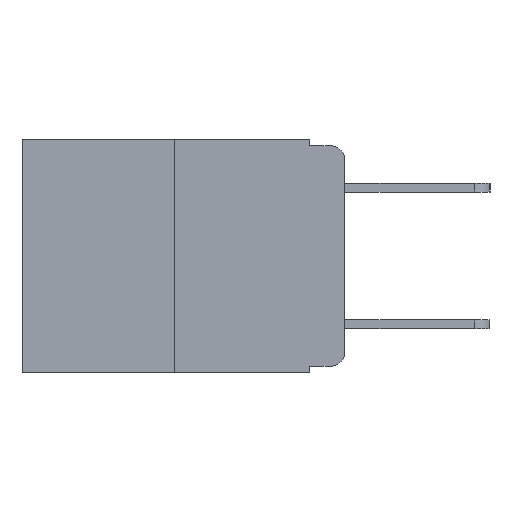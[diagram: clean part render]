
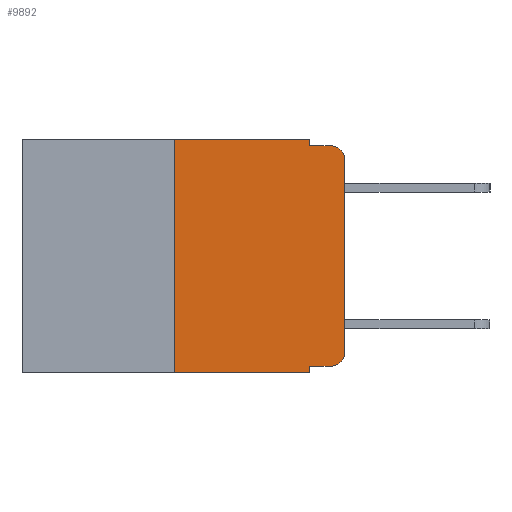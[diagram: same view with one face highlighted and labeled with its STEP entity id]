
A CAD part, left-side view. The second image highlights one B-rep face of the part: STEP entity #9892.
In plain terms, the highlighted planar face has unit normal (-1, 0, 0).
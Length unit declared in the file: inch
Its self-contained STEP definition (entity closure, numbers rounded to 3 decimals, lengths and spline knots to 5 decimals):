
#5 = DIRECTION ( 'NONE',  ( -1., 0., 0. ) ) ;
#24 = LINE ( 'NONE', #9948, #9604 ) ;
#371 = ORIENTED_EDGE ( 'NONE', *, *, #2360, .T. ) ;
#423 = CARTESIAN_POINT ( 'NONE',  ( 0., 0.051, -0.01 ) ) ;
#494 = VERTEX_POINT ( 'NONE', #6020 ) ;
#500 = LINE ( 'NONE', #2824, #9484 ) ;
#669 = VERTEX_POINT ( 'NONE', #9524 ) ;
#785 = LINE ( 'NONE', #10583, #5287 ) ;
#791 = CARTESIAN_POINT ( 'NONE',  ( 0., 0.25, 0. ) ) ;
#915 = VERTEX_POINT ( 'NONE', #4811 ) ;
#1352 = EDGE_CURVE ( 'NONE', #6785, #8225, #785, .T. ) ;
#1600 = EDGE_CURVE ( 'NONE', #3743, #2445, #8336, .T. ) ;
#1873 = ORIENTED_EDGE ( 'NONE', *, *, #1600, .T. ) ;
#1951 = DIRECTION ( 'NONE',  ( 0., -1., 0. ) ) ;
#1996 = CARTESIAN_POINT ( 'NONE',  ( 0., 0.051, -0.333 ) ) ;
#2031 = VERTEX_POINT ( 'NONE', #7292 ) ;
#2129 = LINE ( 'NONE', #4757, #11149 ) ;
#2158 = ORIENTED_EDGE ( 'NONE', *, *, #7004, .T. ) ;
#2360 = EDGE_CURVE ( 'NONE', #2031, #915, #2129, .T. ) ;
#2445 = VERTEX_POINT ( 'NONE', #4334 ) ;
#2824 = CARTESIAN_POINT ( 'NONE',  ( 0., 0., 0. ) ) ;
#2849 = EDGE_CURVE ( 'NONE', #669, #7589, #500, .T. ) ;
#3039 = DIRECTION ( 'NONE',  ( 0., 0., 1. ) ) ;
#3146 = DIRECTION ( 'NONE',  ( 0., -1., 0. ) ) ;
#3434 = ORIENTED_EDGE ( 'NONE', *, *, #6601, .F. ) ;
#3544 = PLANE ( 'NONE',  #4599 ) ;
#3712 = EDGE_LOOP ( 'NONE', ( #5486, #8665, #9512, #7982, #3840, #4403, #371, #3434, #1873, #2158 ) ) ;
#3743 = VERTEX_POINT ( 'NONE', #6516 ) ;
#3840 = ORIENTED_EDGE ( 'NONE', *, *, #3918, .F. ) ;
#3918 = EDGE_CURVE ( 'NONE', #494, #6785, #24, .T. ) ;
#3938 = CARTESIAN_POINT ( 'NONE',  ( 0., 0.051, 0. ) ) ;
#4020 = LINE ( 'NONE', #791, #8420 ) ;
#4027 = CIRCLE ( 'NONE', #5979, 0.02 ) ;
#4334 = CARTESIAN_POINT ( 'NONE',  ( 0., 0.02, -0.333 ) ) ;
#4403 = ORIENTED_EDGE ( 'NONE', *, *, #7378, .F. ) ;
#4441 = DIRECTION ( 'NONE',  ( 1., 0., 0. ) ) ;
#4599 = AXIS2_PLACEMENT_3D ( 'NONE', #11319, #4441, #10545 ) ;
#4757 = CARTESIAN_POINT ( 'NONE',  ( 0., 0.473, -0.343 ) ) ;
#4811 = CARTESIAN_POINT ( 'NONE',  ( 0., 0.051, -0.343 ) ) ;
#5054 = CARTESIAN_POINT ( 'NONE',  ( 0., 0.02, -0.03 ) ) ;
#5068 = FACE_OUTER_BOUND ( 'NONE', #3712, .T. ) ;
#5287 = VECTOR ( 'NONE', #7171, 39.37008 ) ;
#5456 = AXIS2_PLACEMENT_3D ( 'NONE', #5054, #11115, #5936 ) ;
#5457 = CARTESIAN_POINT ( 'NONE',  ( 0., 0.02, -0.313 ) ) ;
#5486 = ORIENTED_EDGE ( 'NONE', *, *, #2849, .T. ) ;
#5913 = VERTEX_POINT ( 'NONE', #9069 ) ;
#5936 = DIRECTION ( 'NONE',  ( 0., 0., -1. ) ) ;
#5979 = AXIS2_PLACEMENT_3D ( 'NONE', #5457, #5, #6356 ) ;
#6020 = CARTESIAN_POINT ( 'NONE',  ( 0., 0.25, 0. ) ) ;
#6171 = EDGE_CURVE ( 'NONE', #7589, #5913, #10599, .T. ) ;
#6356 = DIRECTION ( 'NONE',  ( 0., 0., -1. ) ) ;
#6516 = CARTESIAN_POINT ( 'NONE',  ( 0., 0.051, -0.333 ) ) ;
#6601 = EDGE_CURVE ( 'NONE', #3743, #915, #9007, .T. ) ;
#6785 = VERTEX_POINT ( 'NONE', #9536 ) ;
#7004 = EDGE_CURVE ( 'NONE', #2445, #669, #4027, .T. ) ;
#7171 = DIRECTION ( 'NONE',  ( 0., 0., -1. ) ) ;
#7292 = CARTESIAN_POINT ( 'NONE',  ( 0., 0.25, -0.343 ) ) ;
#7378 = EDGE_CURVE ( 'NONE', #2031, #494, #4020, .T. ) ;
#7585 = LINE ( 'NONE', #423, #10172 ) ;
#7589 = VERTEX_POINT ( 'NONE', #10127 ) ;
#7642 = DIRECTION ( 'NONE',  ( 0., -1., 0. ) ) ;
#7799 = CARTESIAN_POINT ( 'NONE',  ( 0., 0.051, -0.01 ) ) ;
#7982 = ORIENTED_EDGE ( 'NONE', *, *, #1352, .F. ) ;
#8153 = EDGE_CURVE ( 'NONE', #8225, #5913, #7585, .T. ) ;
#8225 = VERTEX_POINT ( 'NONE', #7799 ) ;
#8336 = LINE ( 'NONE', #1996, #10380 ) ;
#8420 = VECTOR ( 'NONE', #10529, 39.37008 ) ;
#8665 = ORIENTED_EDGE ( 'NONE', *, *, #6171, .T. ) ;
#8720 = VECTOR ( 'NONE', #9230, 39.37008 ) ;
#9007 = LINE ( 'NONE', #3938, #8720 ) ;
#9069 = CARTESIAN_POINT ( 'NONE',  ( 0., 0.02, -0.01 ) ) ;
#9230 = DIRECTION ( 'NONE',  ( 0., 0., -1. ) ) ;
#9443 = DIRECTION ( 'NONE',  ( 0., -1., 0. ) ) ;
#9484 = VECTOR ( 'NONE', #3039, 39.37008 ) ;
#9512 = ORIENTED_EDGE ( 'NONE', *, *, #8153, .F. ) ;
#9524 = CARTESIAN_POINT ( 'NONE',  ( 0., 0., -0.313 ) ) ;
#9536 = CARTESIAN_POINT ( 'NONE',  ( 0., 0.051, 0. ) ) ;
#9604 = VECTOR ( 'NONE', #3146, 39.37008 ) ;
#9892 = ADVANCED_FACE ( 'NONE', ( #5068 ), #3544, .F. ) ;
#9948 = CARTESIAN_POINT ( 'NONE',  ( 0., 0.473, 0. ) ) ;
#10127 = CARTESIAN_POINT ( 'NONE',  ( 0., 0., -0.03 ) ) ;
#10172 = VECTOR ( 'NONE', #7642, 39.37008 ) ;
#10380 = VECTOR ( 'NONE', #1951, 39.37008 ) ;
#10529 = DIRECTION ( 'NONE',  ( 0., 0., 1. ) ) ;
#10545 = DIRECTION ( 'NONE',  ( 0., 0., -1. ) ) ;
#10583 = CARTESIAN_POINT ( 'NONE',  ( 0., 0.051, 0. ) ) ;
#10599 = CIRCLE ( 'NONE', #5456, 0.02 ) ;
#11115 = DIRECTION ( 'NONE',  ( -1., 0., 0. ) ) ;
#11149 = VECTOR ( 'NONE', #9443, 39.37008 ) ;
#11319 = CARTESIAN_POINT ( 'NONE',  ( 0., 0.473, 0. ) ) ;
